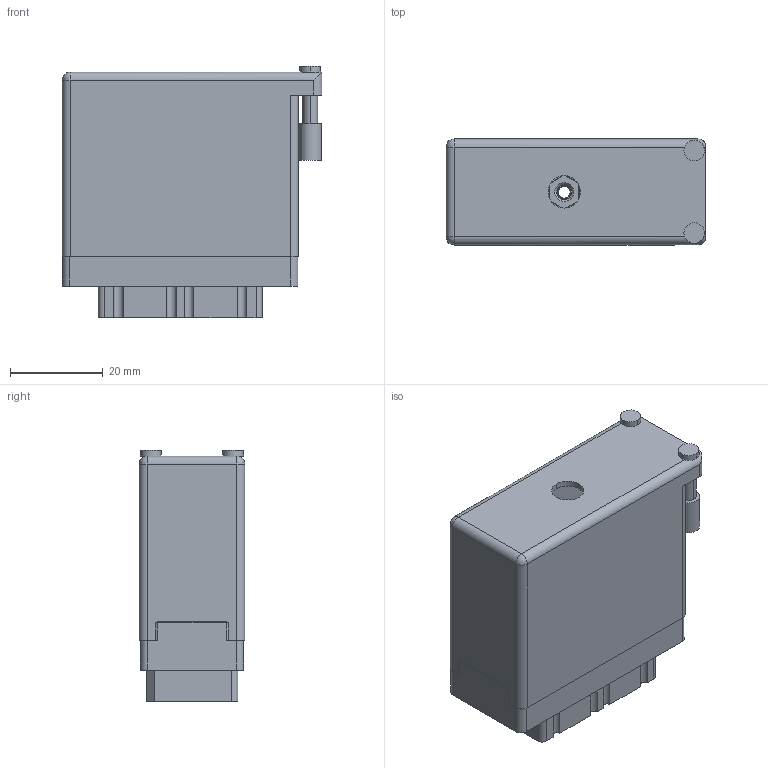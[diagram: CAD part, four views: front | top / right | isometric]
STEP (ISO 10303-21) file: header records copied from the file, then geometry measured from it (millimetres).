
FILE_DESCRIPTION (( 'STEP AP203' ), '1' );
FILE_NAME ('519-036-000-456.STEP', '2020-09-09T20:05:30', ( '' ), ( '' ), 'SwSTEP 2.0', 'SolidWorks 2020', '' );
FILE_SCHEMA (( 'CONFIG_CONTROL_DESIGN' ));
Length unit declared in the file: inch
Products named in the file (4): 519 Receptacle Insulator_036; 519-036-000-456; 516-230-001_Metal - 038 Side Entry; 516-252-035-100_516-252-035-100
Assembly tree (3 placements, depth 2):
  519-036-000-456
    519 Receptacle Insulator_036
    516-252-035-100_516-252-035-100
    516-230-001_Metal - 038 Side Entry
Bounding box: 56.08 x 22.83 x 54.28 mm (x, y, z)
Volume: 20030.9 mm3; surface area: 27946.9 mm2
Topology: 3 solids, 3 shells, 962 faces, 2788 edges, 1850 vertices
Faces by surface type: plane 655, cylinder 287, cone 12, bspline 6, sphere 2
Entity records: 34588 total; most frequent: CARTESIAN_POINT 8091, ORIENTED_EDGE 5572, DIRECTION 5358, EDGE_CURVE 2786, LINE 2028, VECTOR 2028, VERTEX_POINT 1850, AXIS2_PLACEMENT_3D 1665
